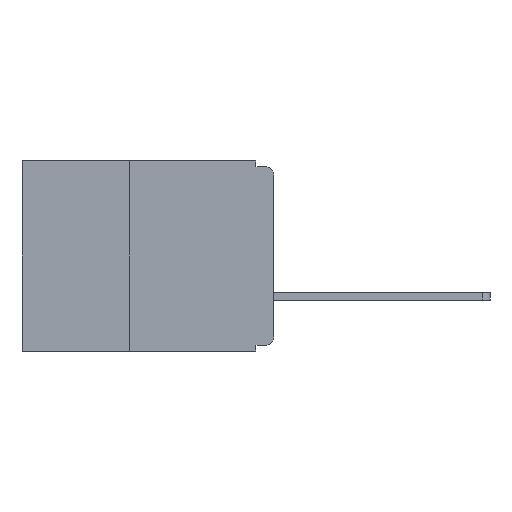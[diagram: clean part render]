
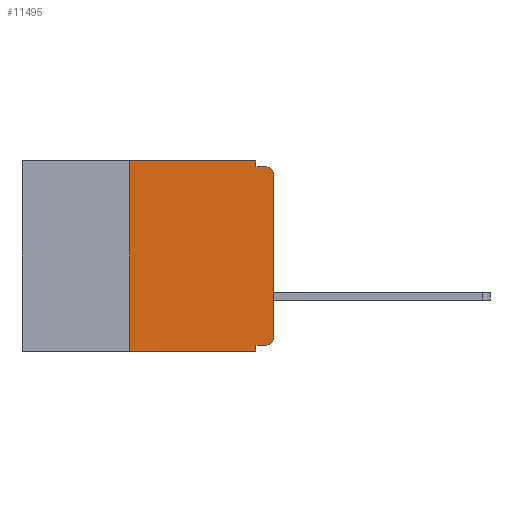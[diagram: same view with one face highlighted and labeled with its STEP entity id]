
A CAD part, left-side view. The second image highlights one B-rep face of the part: STEP entity #11495.
In plain terms, the highlighted planar face has unit normal (-1, 0, 0).
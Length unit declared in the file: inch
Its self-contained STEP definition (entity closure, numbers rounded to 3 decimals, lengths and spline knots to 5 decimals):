
#345 = VERTEX_POINT ( 'NONE', #27477 ) ;
#528 = EDGE_CURVE ( 'NONE', #9814, #28473, #13474, .T. ) ;
#864 = ORIENTED_EDGE ( 'NONE', *, *, #13579, .F. ) ;
#1022 = DIRECTION ( 'NONE',  ( 0., 0., -1. ) ) ;
#1046 = VECTOR ( 'NONE', #28499, 39.37008 ) ;
#1545 = CARTESIAN_POINT ( 'NONE',  ( 0., 0.031, 0. ) ) ;
#1859 = CARTESIAN_POINT ( 'NONE',  ( 0., 0., -0.01 ) ) ;
#2936 = CARTESIAN_POINT ( 'NONE',  ( 0., 0.031, -0.01 ) ) ;
#3378 = VERTEX_POINT ( 'NONE', #14166 ) ;
#3464 = DIRECTION ( 'NONE',  ( 0., 0., 1. ) ) ;
#3819 = VERTEX_POINT ( 'NONE', #20039 ) ;
#4087 = VERTEX_POINT ( 'NONE', #9330 ) ;
#4231 = VERTEX_POINT ( 'NONE', #2936 ) ;
#4504 = DIRECTION ( 'NONE',  ( 0., -1., 0. ) ) ;
#5196 = ORIENTED_EDGE ( 'NONE', *, *, #30312, .T. ) ;
#5984 = DIRECTION ( 'NONE',  ( 0., -1., 0. ) ) ;
#6925 = ORIENTED_EDGE ( 'NONE', *, *, #21144, .F. ) ;
#8013 = LINE ( 'NONE', #10830, #1046 ) ;
#8407 = AXIS2_PLACEMENT_3D ( 'NONE', #24011, #16604, #1022 ) ;
#8664 = EDGE_CURVE ( 'NONE', #4087, #4231, #28355, .T. ) ;
#9159 = EDGE_CURVE ( 'NONE', #15378, #4087, #14664, .T. ) ;
#9329 = EDGE_LOOP ( 'NONE', ( #15775, #32078, #6925, #31885, #10068, #10805, #5196, #864, #27870, #21724 ) ) ;
#9330 = CARTESIAN_POINT ( 'NONE',  ( 0., 0.031, 0. ) ) ;
#9443 = LINE ( 'NONE', #20235, #14716 ) ;
#9751 = VECTOR ( 'NONE', #19628, 39.37008 ) ;
#9814 = VERTEX_POINT ( 'NONE', #22168 ) ;
#10068 = ORIENTED_EDGE ( 'NONE', *, *, #9159, .F. ) ;
#10610 = CARTESIAN_POINT ( 'NONE',  ( 0., 0.25, -0.33 ) ) ;
#10805 = ORIENTED_EDGE ( 'NONE', *, *, #19688, .F. ) ;
#10830 = CARTESIAN_POINT ( 'NONE',  ( 0., 0.25, -0.33 ) ) ;
#11495 = ADVANCED_FACE ( 'NONE', ( #30847 ), #31466, .F. ) ;
#11514 = LINE ( 'NONE', #28169, #24178 ) ;
#11552 = VECTOR ( 'NONE', #3464, 39.37008 ) ;
#12749 = LINE ( 'NONE', #32436, #24570 ) ;
#12979 = DIRECTION ( 'NONE',  ( -1., 0., 0. ) ) ;
#13132 = AXIS2_PLACEMENT_3D ( 'NONE', #28038, #12979, #30496 ) ;
#13474 = CIRCLE ( 'NONE', #15105, 0.015 ) ;
#13579 = EDGE_CURVE ( 'NONE', #345, #3819, #12749, .T. ) ;
#13804 = CARTESIAN_POINT ( 'NONE',  ( 0., 0.437, 0. ) ) ;
#14166 = CARTESIAN_POINT ( 'NONE',  ( 0., 0., -0.305 ) ) ;
#14664 = LINE ( 'NONE', #13804, #27189 ) ;
#14716 = VECTOR ( 'NONE', #25229, 39.37008 ) ;
#14917 = VERTEX_POINT ( 'NONE', #18305 ) ;
#15105 = AXIS2_PLACEMENT_3D ( 'NONE', #15333, #15328, #15217 ) ;
#15217 = DIRECTION ( 'NONE',  ( 0., 0., -1. ) ) ;
#15328 = DIRECTION ( 'NONE',  ( -1., 0., 0. ) ) ;
#15333 = CARTESIAN_POINT ( 'NONE',  ( 0., 0.015, -0.025 ) ) ;
#15378 = VERTEX_POINT ( 'NONE', #22608 ) ;
#15775 = ORIENTED_EDGE ( 'NONE', *, *, #29872, .T. ) ;
#16009 = LINE ( 'NONE', #1859, #21878 ) ;
#16604 = DIRECTION ( 'NONE',  ( 1., 0., 0. ) ) ;
#16683 = CARTESIAN_POINT ( 'NONE',  ( 0., 0.015, -0.01 ) ) ;
#17580 = EDGE_CURVE ( 'NONE', #14917, #3378, #27607, .T. ) ;
#18305 = CARTESIAN_POINT ( 'NONE',  ( 0., 0.015, -0.32 ) ) ;
#19628 = DIRECTION ( 'NONE',  ( 0., 0., -1. ) ) ;
#19688 = EDGE_CURVE ( 'NONE', #23938, #15378, #8013, .T. ) ;
#20039 = CARTESIAN_POINT ( 'NONE',  ( 0., 0.031, -0.33 ) ) ;
#20235 = CARTESIAN_POINT ( 'NONE',  ( 0., 0., -0.32 ) ) ;
#21144 = EDGE_CURVE ( 'NONE', #4231, #28473, #16009, .T. ) ;
#21437 = CARTESIAN_POINT ( 'NONE',  ( 0., 0., 0. ) ) ;
#21724 = ORIENTED_EDGE ( 'NONE', *, *, #17580, .T. ) ;
#21878 = VECTOR ( 'NONE', #4504, 39.37008 ) ;
#22168 = CARTESIAN_POINT ( 'NONE',  ( 0., 0., -0.025 ) ) ;
#22608 = CARTESIAN_POINT ( 'NONE',  ( 0., 0.25, 0. ) ) ;
#23785 = EDGE_CURVE ( 'NONE', #14917, #345, #9443, .T. ) ;
#23938 = VERTEX_POINT ( 'NONE', #10610 ) ;
#24011 = CARTESIAN_POINT ( 'NONE',  ( 0., 0.437, 0. ) ) ;
#24178 = VECTOR ( 'NONE', #30609, 39.37008 ) ;
#24570 = VECTOR ( 'NONE', #27511, 39.37008 ) ;
#25229 = DIRECTION ( 'NONE',  ( 0., 1., 0. ) ) ;
#27189 = VECTOR ( 'NONE', #5984, 39.37008 ) ;
#27477 = CARTESIAN_POINT ( 'NONE',  ( 0., 0.031, -0.32 ) ) ;
#27511 = DIRECTION ( 'NONE',  ( 0., 0., -1. ) ) ;
#27607 = CIRCLE ( 'NONE', #13132, 0.015 ) ;
#27870 = ORIENTED_EDGE ( 'NONE', *, *, #23785, .F. ) ;
#28038 = CARTESIAN_POINT ( 'NONE',  ( 0., 0.015, -0.305 ) ) ;
#28169 = CARTESIAN_POINT ( 'NONE',  ( 0., 0.437, -0.33 ) ) ;
#28355 = LINE ( 'NONE', #1545, #9751 ) ;
#28473 = VERTEX_POINT ( 'NONE', #16683 ) ;
#28499 = DIRECTION ( 'NONE',  ( 0., 0., 1. ) ) ;
#29872 = EDGE_CURVE ( 'NONE', #3378, #9814, #31554, .T. ) ;
#30312 = EDGE_CURVE ( 'NONE', #23938, #3819, #11514, .T. ) ;
#30496 = DIRECTION ( 'NONE',  ( 0., 0., -1. ) ) ;
#30609 = DIRECTION ( 'NONE',  ( 0., -1., 0. ) ) ;
#30847 = FACE_OUTER_BOUND ( 'NONE', #9329, .T. ) ;
#31466 = PLANE ( 'NONE',  #8407 ) ;
#31554 = LINE ( 'NONE', #21437, #11552 ) ;
#31885 = ORIENTED_EDGE ( 'NONE', *, *, #8664, .F. ) ;
#32078 = ORIENTED_EDGE ( 'NONE', *, *, #528, .T. ) ;
#32436 = CARTESIAN_POINT ( 'NONE',  ( 0., 0.031, -0.33 ) ) ;
